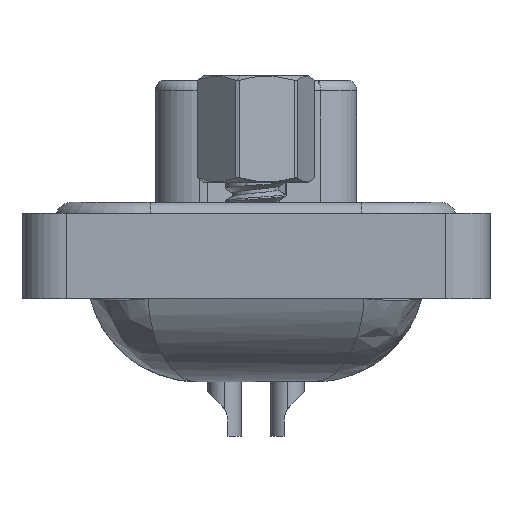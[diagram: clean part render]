
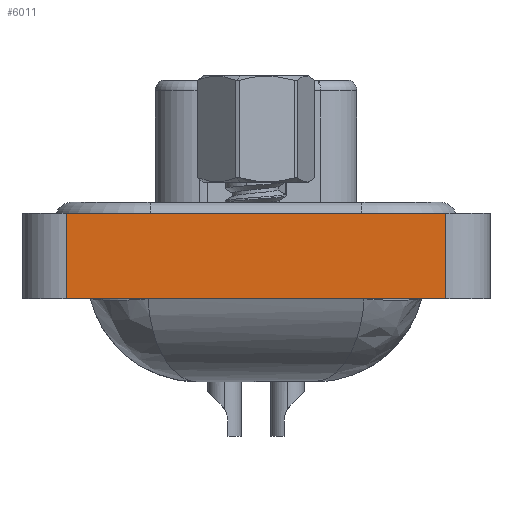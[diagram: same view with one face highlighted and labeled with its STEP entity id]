
A CAD part, left-side view. The second image highlights one B-rep face of the part: STEP entity #6011.
In plain terms, the highlighted planar face has unit normal (-1, 0, 0).
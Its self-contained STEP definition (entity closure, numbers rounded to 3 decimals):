
#356 = CARTESIAN_POINT ( 'NONE',  ( -7.15, 8.55, 0.5 ) ) ;
#1125 = CARTESIAN_POINT ( 'NONE',  ( -7.15, -8.55, -3.35 ) ) ;
#4412 = LINE ( 'NONE', #14686, #14954 ) ;
#4828 = EDGE_LOOP ( 'NONE', ( #6053, #30286, #12247, #20963 ) ) ;
#6011 = ADVANCED_FACE ( 'NONE', ( #20942 ), #15917, .T. ) ;
#6053 = ORIENTED_EDGE ( 'NONE', *, *, #31921, .T. ) ;
#6454 = LINE ( 'NONE', #31341, #31121 ) ;
#6495 = VECTOR ( 'NONE', #26725, 1000. ) ;
#11988 = DIRECTION ( 'NONE',  ( 0., -1., 0. ) ) ;
#12247 = ORIENTED_EDGE ( 'NONE', *, *, #29458, .F. ) ;
#12719 = DIRECTION ( 'NONE',  ( -1., 0., 0. ) ) ;
#13283 = LINE ( 'NONE', #21017, #6495 ) ;
#13377 = CARTESIAN_POINT ( 'NONE',  ( -7.15, -8.55, -3.35 ) ) ;
#14686 = CARTESIAN_POINT ( 'NONE',  ( -7.15, -8.55, 0.5 ) ) ;
#14954 = VECTOR ( 'NONE', #19556, 1000. ) ;
#15917 = PLANE ( 'NONE',  #30078 ) ;
#16269 = CARTESIAN_POINT ( 'NONE',  ( -7.15, 8.55, -3.35 ) ) ;
#18914 = DIRECTION ( 'NONE',  ( 0., 0., 1. ) ) ;
#19556 = DIRECTION ( 'NONE',  ( 0., -1., 0. ) ) ;
#20458 = DIRECTION ( 'NONE',  ( 0., 0., 1. ) ) ;
#20942 = FACE_OUTER_BOUND ( 'NONE', #4828, .T. ) ;
#20963 = ORIENTED_EDGE ( 'NONE', *, *, #27899, .T. ) ;
#21017 = CARTESIAN_POINT ( 'NONE',  ( -7.15, 8.55, -3.35 ) ) ;
#21875 = LINE ( 'NONE', #32119, #24124 ) ;
#22117 = VERTEX_POINT ( 'NONE', #356 ) ;
#24061 = VERTEX_POINT ( 'NONE', #16269 ) ;
#24124 = VECTOR ( 'NONE', #11988, 1000. ) ;
#26407 = EDGE_CURVE ( 'NONE', #22117, #29276, #4412, .T. ) ;
#26725 = DIRECTION ( 'NONE',  ( 0., 0., 1. ) ) ;
#27771 = CARTESIAN_POINT ( 'NONE',  ( -7.15, -8.55, 0.5 ) ) ;
#27899 = EDGE_CURVE ( 'NONE', #24061, #31422, #21875, .T. ) ;
#29276 = VERTEX_POINT ( 'NONE', #27771 ) ;
#29458 = EDGE_CURVE ( 'NONE', #24061, #22117, #13283, .T. ) ;
#30078 = AXIS2_PLACEMENT_3D ( 'NONE', #13377, #12719, #20458 ) ;
#30286 = ORIENTED_EDGE ( 'NONE', *, *, #26407, .F. ) ;
#31121 = VECTOR ( 'NONE', #18914, 1000. ) ;
#31341 = CARTESIAN_POINT ( 'NONE',  ( -7.15, -8.55, -3.35 ) ) ;
#31422 = VERTEX_POINT ( 'NONE', #1125 ) ;
#31921 = EDGE_CURVE ( 'NONE', #31422, #29276, #6454, .T. ) ;
#32119 = CARTESIAN_POINT ( 'NONE',  ( -7.15, -8.55, -3.35 ) ) ;
